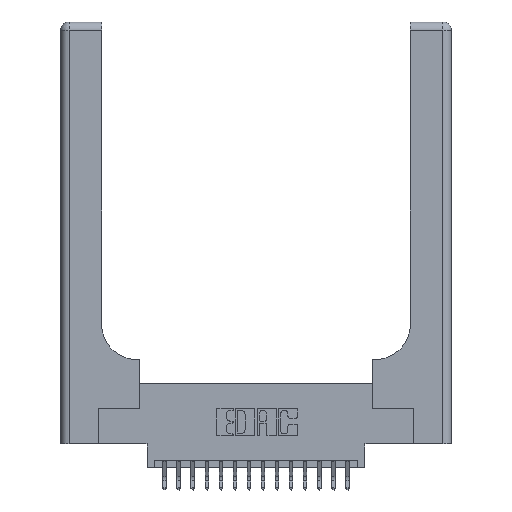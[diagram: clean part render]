
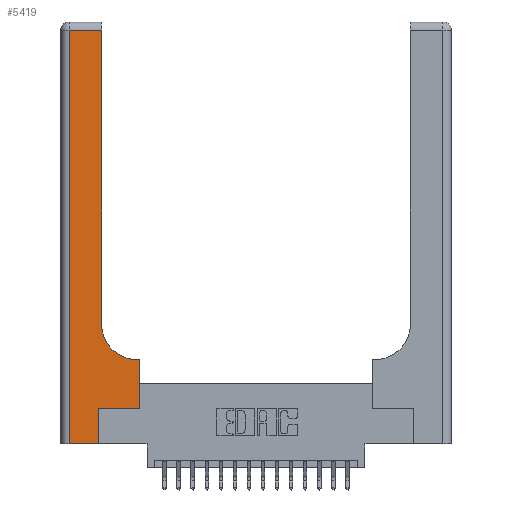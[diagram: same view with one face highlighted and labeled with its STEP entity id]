
A CAD part, top view. The second image highlights one B-rep face of the part: STEP entity #5419.
In plain terms, the highlighted planar face has unit normal (0, 0, 1).
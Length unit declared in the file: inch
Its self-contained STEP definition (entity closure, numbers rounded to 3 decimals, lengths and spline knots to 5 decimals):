
#142 = ORIENTED_EDGE ( 'NONE', *, *, #6181, .T. ) ;
#153 = VECTOR ( 'NONE', #12805, 39.37008 ) ;
#667 = DIRECTION ( 'NONE',  ( -1., 0., 0. ) ) ;
#1110 = DIRECTION ( 'NONE',  ( 0., 0., -1. ) ) ;
#1395 = CARTESIAN_POINT ( 'NONE',  ( 0.5585, 0.25, 0.37 ) ) ;
#1697 = VERTEX_POINT ( 'NONE', #4106 ) ;
#1839 = LINE ( 'NONE', #4119, #4049 ) ;
#1965 = CARTESIAN_POINT ( 'NONE',  ( 0.269, 0.25, 0.37 ) ) ;
#2410 = DIRECTION ( 'NONE',  ( 0., 1., 0. ) ) ;
#2798 = VECTOR ( 'NONE', #15926, 39.37008 ) ;
#2865 = VERTEX_POINT ( 'NONE', #7703 ) ;
#2880 = CARTESIAN_POINT ( 'NONE',  ( 0.5585, 0.6, 0.37 ) ) ;
#3111 = CARTESIAN_POINT ( 'NONE',  ( 0.2915, 3., 0.37 ) ) ;
#3915 = VERTEX_POINT ( 'NONE', #14790 ) ;
#4049 = VECTOR ( 'NONE', #2410, 39.37008 ) ;
#4096 = PLANE ( 'NONE',  #15456 ) ;
#4106 = CARTESIAN_POINT ( 'NONE',  ( 0.06, 0., 0.37 ) ) ;
#4119 = CARTESIAN_POINT ( 'NONE',  ( 0.5585, 0.25, 0.37 ) ) ;
#4128 = EDGE_CURVE ( 'NONE', #5708, #14619, #9722, .T. ) ;
#5419 = ADVANCED_FACE ( 'NONE', ( #12351 ), #4096, .F. ) ;
#5583 = ORIENTED_EDGE ( 'NONE', *, *, #11277, .T. ) ;
#5605 = VECTOR ( 'NONE', #667, 39.37008 ) ;
#5625 = CARTESIAN_POINT ( 'NONE',  ( 0.269, 0.25, 0.37 ) ) ;
#5673 = LINE ( 'NONE', #18867, #14265 ) ;
#5708 = VERTEX_POINT ( 'NONE', #2880 ) ;
#6181 = EDGE_CURVE ( 'NONE', #18066, #1697, #5673, .T. ) ;
#7703 = CARTESIAN_POINT ( 'NONE',  ( 0.269, 0., 0.37 ) ) ;
#7823 = CARTESIAN_POINT ( 'NONE',  ( 0., 0., 0.37 ) ) ;
#8197 = EDGE_CURVE ( 'NONE', #13157, #3915, #14462, .T. ) ;
#8277 = EDGE_LOOP ( 'NONE', ( #19267, #16096, #142, #5583, #8705, #17095, #12742, #16889, #11782 ) ) ;
#8402 = EDGE_CURVE ( 'NONE', #3915, #18066, #20320, .T. ) ;
#8705 = ORIENTED_EDGE ( 'NONE', *, *, #13933, .T. ) ;
#9448 = DIRECTION ( 'NONE',  ( 0., 0., -1. ) ) ;
#9722 = LINE ( 'NONE', #19391, #5605 ) ;
#9771 = EDGE_CURVE ( 'NONE', #14619, #13157, #14142, .T. ) ;
#10359 = AXIS2_PLACEMENT_3D ( 'NONE', #14019, #9448, #16691 ) ;
#10721 = LINE ( 'NONE', #12739, #153 ) ;
#11104 = DIRECTION ( 'NONE',  ( 0., 1., 0. ) ) ;
#11277 = EDGE_CURVE ( 'NONE', #1697, #2865, #15792, .T. ) ;
#11782 = ORIENTED_EDGE ( 'NONE', *, *, #9771, .T. ) ;
#12351 = FACE_OUTER_BOUND ( 'NONE', #8277, .T. ) ;
#12739 = CARTESIAN_POINT ( 'NONE',  ( 0.269, 0., 0.37 ) ) ;
#12742 = ORIENTED_EDGE ( 'NONE', *, *, #15226, .T. ) ;
#12805 = DIRECTION ( 'NONE',  ( 0., 1., 0. ) ) ;
#13157 = VERTEX_POINT ( 'NONE', #18753 ) ;
#13612 = VECTOR ( 'NONE', #15111, 39.37008 ) ;
#13663 = VERTEX_POINT ( 'NONE', #1395 ) ;
#13933 = EDGE_CURVE ( 'NONE', #2865, #15984, #10721, .T. ) ;
#14019 = CARTESIAN_POINT ( 'NONE',  ( 0.5415, 0.85, 0.37 ) ) ;
#14142 = CIRCLE ( 'NONE', #10359, 0.25 ) ;
#14227 = VECTOR ( 'NONE', #11104, 39.37008 ) ;
#14265 = VECTOR ( 'NONE', #18661, 39.37008 ) ;
#14462 = LINE ( 'NONE', #3111, #14227 ) ;
#14619 = VERTEX_POINT ( 'NONE', #17909 ) ;
#14790 = CARTESIAN_POINT ( 'NONE',  ( 0.2915, 2.94, 0.37 ) ) ;
#14794 = CARTESIAN_POINT ( 'NONE',  ( 0., 2.94, 0.37 ) ) ;
#15111 = DIRECTION ( 'NONE',  ( 1., 0., 0. ) ) ;
#15226 = EDGE_CURVE ( 'NONE', #13663, #5708, #1839, .T. ) ;
#15456 = AXIS2_PLACEMENT_3D ( 'NONE', #18314, #1110, #17267 ) ;
#15740 = EDGE_CURVE ( 'NONE', #15984, #13663, #17772, .T. ) ;
#15792 = LINE ( 'NONE', #7823, #2798 ) ;
#15926 = DIRECTION ( 'NONE',  ( 1., 0., 0. ) ) ;
#15984 = VERTEX_POINT ( 'NONE', #5625 ) ;
#16096 = ORIENTED_EDGE ( 'NONE', *, *, #8402, .T. ) ;
#16172 = VECTOR ( 'NONE', #19218, 39.37008 ) ;
#16237 = CARTESIAN_POINT ( 'NONE',  ( 0.06, 2.94, 0.37 ) ) ;
#16691 = DIRECTION ( 'NONE',  ( 1., 0., 0. ) ) ;
#16889 = ORIENTED_EDGE ( 'NONE', *, *, #4128, .T. ) ;
#17095 = ORIENTED_EDGE ( 'NONE', *, *, #15740, .T. ) ;
#17267 = DIRECTION ( 'NONE',  ( -1., 0., 0. ) ) ;
#17772 = LINE ( 'NONE', #1965, #13612 ) ;
#17909 = CARTESIAN_POINT ( 'NONE',  ( 0.5415, 0.6, 0.37 ) ) ;
#18066 = VERTEX_POINT ( 'NONE', #16237 ) ;
#18314 = CARTESIAN_POINT ( 'NONE',  ( 0., 3., 0.37 ) ) ;
#18661 = DIRECTION ( 'NONE',  ( 0., -1., 0. ) ) ;
#18753 = CARTESIAN_POINT ( 'NONE',  ( 0.2915, 0.85, 0.37 ) ) ;
#18867 = CARTESIAN_POINT ( 'NONE',  ( 0.06, 3., 0.37 ) ) ;
#19218 = DIRECTION ( 'NONE',  ( -1., 0., 0. ) ) ;
#19267 = ORIENTED_EDGE ( 'NONE', *, *, #8197, .T. ) ;
#19391 = CARTESIAN_POINT ( 'NONE',  ( 0.2915, 0.6, 0.37 ) ) ;
#20320 = LINE ( 'NONE', #14794, #16172 ) ;
